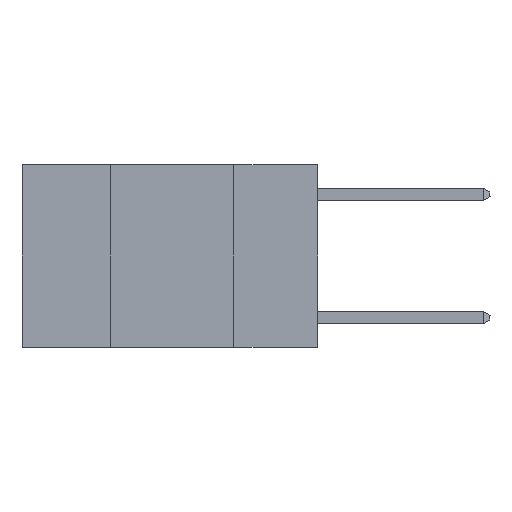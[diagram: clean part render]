
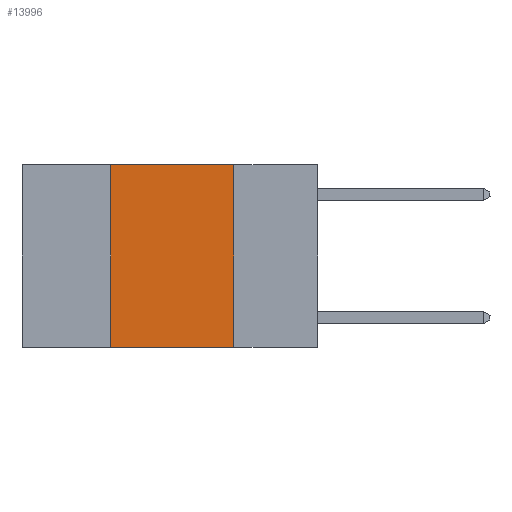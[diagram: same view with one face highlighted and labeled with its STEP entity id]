
A CAD part, left-side view. The second image highlights one B-rep face of the part: STEP entity #13996.
In plain terms, the highlighted planar face has unit normal (-1, 0, 0).
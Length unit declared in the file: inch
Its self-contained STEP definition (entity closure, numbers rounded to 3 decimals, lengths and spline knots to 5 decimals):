
#447 = VECTOR ( 'NONE', #11102, 39.37008 ) ;
#1292 = CARTESIAN_POINT ( 'NONE',  ( 0., 0.17, 0. ) ) ;
#1598 = CARTESIAN_POINT ( 'NONE',  ( 0., 0.6, 0. ) ) ;
#1623 = CARTESIAN_POINT ( 'NONE',  ( 0., 0.6, 0. ) ) ;
#1684 = DIRECTION ( 'NONE',  ( 0., -1., 0. ) ) ;
#2083 = VECTOR ( 'NONE', #9978, 39.37008 ) ;
#2537 = ORIENTED_EDGE ( 'NONE', *, *, #13766, .F. ) ;
#2783 = AXIS2_PLACEMENT_3D ( 'NONE', #1623, #7034, #11510 ) ;
#3503 = VECTOR ( 'NONE', #1684, 39.37008 ) ;
#3825 = VERTEX_POINT ( 'NONE', #1292 ) ;
#3835 = ORIENTED_EDGE ( 'NONE', *, *, #9708, .T. ) ;
#4637 = VERTEX_POINT ( 'NONE', #4656 ) ;
#4656 = CARTESIAN_POINT ( 'NONE',  ( 0., 0.42, -0.37 ) ) ;
#4894 = FACE_OUTER_BOUND ( 'NONE', #11140, .T. ) ;
#5589 = DIRECTION ( 'NONE',  ( 0., 0., -1. ) ) ;
#6118 = VECTOR ( 'NONE', #5589, 39.37008 ) ;
#7034 = DIRECTION ( 'NONE',  ( 1., 0., 0. ) ) ;
#7148 = LINE ( 'NONE', #1598, #3503 ) ;
#7184 = VERTEX_POINT ( 'NONE', #11248 ) ;
#8123 = PLANE ( 'NONE',  #2783 ) ;
#8630 = CARTESIAN_POINT ( 'NONE',  ( 0., 0.17, 0. ) ) ;
#9048 = CARTESIAN_POINT ( 'NONE',  ( 0., 0.6, -0.37 ) ) ;
#9413 = VERTEX_POINT ( 'NONE', #12735 ) ;
#9500 = EDGE_CURVE ( 'NONE', #9413, #3825, #7148, .T. ) ;
#9708 = EDGE_CURVE ( 'NONE', #4637, #7184, #10186, .T. ) ;
#9872 = CARTESIAN_POINT ( 'NONE',  ( 0., 0.42, 0. ) ) ;
#9933 = EDGE_CURVE ( 'NONE', #4637, #9413, #13233, .T. ) ;
#9934 = ORIENTED_EDGE ( 'NONE', *, *, #9933, .F. ) ;
#9978 = DIRECTION ( 'NONE',  ( 0., -1., 0. ) ) ;
#10186 = LINE ( 'NONE', #9048, #2083 ) ;
#11102 = DIRECTION ( 'NONE',  ( 0., 0., 1. ) ) ;
#11140 = EDGE_LOOP ( 'NONE', ( #2537, #12408, #9934, #3835 ) ) ;
#11248 = CARTESIAN_POINT ( 'NONE',  ( 0., 0.17, -0.37 ) ) ;
#11510 = DIRECTION ( 'NONE',  ( 0., 0., -1. ) ) ;
#12408 = ORIENTED_EDGE ( 'NONE', *, *, #9500, .F. ) ;
#12735 = CARTESIAN_POINT ( 'NONE',  ( 0., 0.42, 0. ) ) ;
#13233 = LINE ( 'NONE', #9872, #447 ) ;
#13766 = EDGE_CURVE ( 'NONE', #3825, #7184, #14207, .T. ) ;
#13996 = ADVANCED_FACE ( 'NONE', ( #4894 ), #8123, .F. ) ;
#14207 = LINE ( 'NONE', #8630, #6118 ) ;
